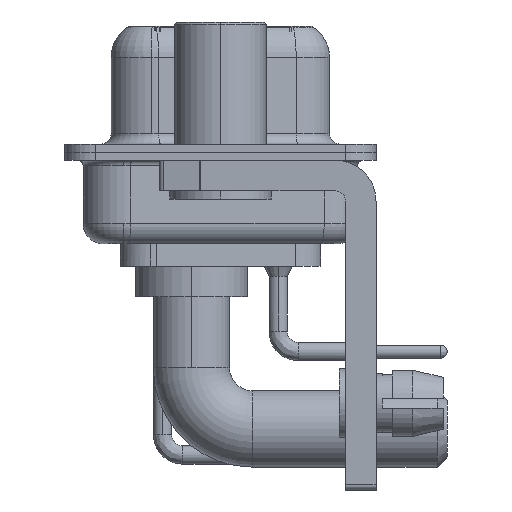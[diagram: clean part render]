
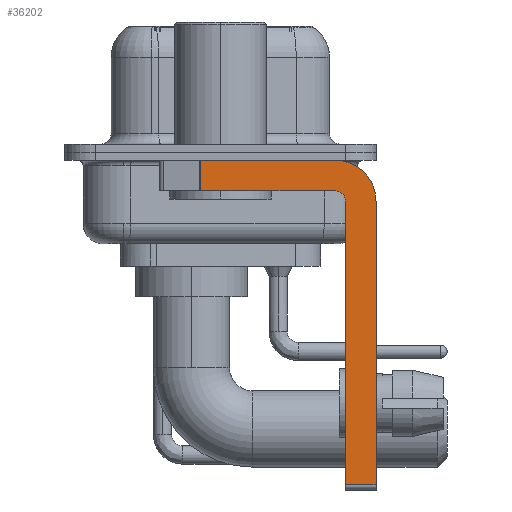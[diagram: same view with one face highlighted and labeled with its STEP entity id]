
A CAD part, left-side view. The second image highlights one B-rep face of the part: STEP entity #36202.
In plain terms, the highlighted planar face has unit normal (-1, 0, 0).
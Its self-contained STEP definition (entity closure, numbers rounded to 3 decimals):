
#147 = ORIENTED_EDGE ( 'NONE', *, *, #24818, .T. ) ;
#672 = VERTEX_POINT ( 'NONE', #22985 ) ;
#847 = DIRECTION ( 'NONE',  ( 0., -1., 0. ) ) ;
#1562 = VERTEX_POINT ( 'NONE', #23226 ) ;
#2220 = DIRECTION ( 'NONE',  ( 0., 0., -1. ) ) ;
#3119 = CARTESIAN_POINT ( 'NONE',  ( -2.9, -5.65, -2.4 ) ) ;
#3368 = CARTESIAN_POINT ( 'NONE',  ( -2.9, -7.65, -2.4 ) ) ;
#3698 = VECTOR ( 'NONE', #24557, 1000. ) ;
#4134 = EDGE_CURVE ( 'NONE', #32855, #33410, #8044, .T. ) ;
#4230 = LINE ( 'NONE', #33460, #3698 ) ;
#4348 = EDGE_CURVE ( 'NONE', #1562, #32855, #32166, .T. ) ;
#4890 = CARTESIAN_POINT ( 'NONE',  ( -2.9, -5.65, -2.4 ) ) ;
#5260 = DIRECTION ( 'NONE',  ( 1., 0., 0. ) ) ;
#5754 = LINE ( 'NONE', #34945, #12010 ) ;
#7094 = DIRECTION ( 'NONE',  ( 0., 0., -1. ) ) ;
#8044 = CIRCLE ( 'NONE', #25629, 2. ) ;
#8614 = EDGE_CURVE ( 'NONE', #25833, #672, #25494, .T. ) ;
#8709 = CARTESIAN_POINT ( 'NONE',  ( -2.9, -5.65, -16.35 ) ) ;
#8791 = DIRECTION ( 'NONE',  ( 0., 0., 1. ) ) ;
#9121 = AXIS2_PLACEMENT_3D ( 'NONE', #3119, #26480, #23445 ) ;
#9213 = CARTESIAN_POINT ( 'NONE',  ( -2.9, 3., -0.4 ) ) ;
#11501 = VECTOR ( 'NONE', #17260, 1000. ) ;
#12010 = VECTOR ( 'NONE', #8791, 1000. ) ;
#12273 = VECTOR ( 'NONE', #847, 1000. ) ;
#12539 = EDGE_LOOP ( 'NONE', ( #29477, #24041, #24917, #35046, #22544, #147, #31158, #20879 ) ) ;
#15218 = CARTESIAN_POINT ( 'NONE',  ( -2.9, -6.15, -2.4 ) ) ;
#15542 = CARTESIAN_POINT ( 'NONE',  ( -2.9, 0.978, -1.9 ) ) ;
#17131 = EDGE_CURVE ( 'NONE', #672, #18011, #26855, .T. ) ;
#17260 = DIRECTION ( 'NONE',  ( 0., -1., 0. ) ) ;
#17402 = EDGE_CURVE ( 'NONE', #26025, #25833, #5754, .T. ) ;
#18011 = VERTEX_POINT ( 'NONE', #15542 ) ;
#18676 = DIRECTION ( 'NONE',  ( 0., 1., 0. ) ) ;
#18722 = VERTEX_POINT ( 'NONE', #28975 ) ;
#19330 = CARTESIAN_POINT ( 'NONE',  ( -2.9, -5.65, -2.4 ) ) ;
#19875 = VECTOR ( 'NONE', #18676, 1000. ) ;
#20879 = ORIENTED_EDGE ( 'NONE', *, *, #4134, .F. ) ;
#21845 = AXIS2_PLACEMENT_3D ( 'NONE', #4890, #5260, #2220 ) ;
#22544 = ORIENTED_EDGE ( 'NONE', *, *, #17402, .F. ) ;
#22985 = CARTESIAN_POINT ( 'NONE',  ( -2.9, -5.65, -1.9 ) ) ;
#23226 = CARTESIAN_POINT ( 'NONE',  ( -2.9, 0.978, -0.4 ) ) ;
#23445 = DIRECTION ( 'NONE',  ( 0., 0., 1. ) ) ;
#23702 = LINE ( 'NONE', #8709, #11501 ) ;
#24041 = ORIENTED_EDGE ( 'NONE', *, *, #37238, .T. ) ;
#24557 = DIRECTION ( 'NONE',  ( 0., 0., -1. ) ) ;
#24818 = EDGE_CURVE ( 'NONE', #26025, #18722, #23702, .T. ) ;
#24917 = ORIENTED_EDGE ( 'NONE', *, *, #17131, .F. ) ;
#25494 = CIRCLE ( 'NONE', #9121, 0.5 ) ;
#25500 = CARTESIAN_POINT ( 'NONE',  ( -2.9, -5.65, -0.4 ) ) ;
#25629 = AXIS2_PLACEMENT_3D ( 'NONE', #19330, #34439, #36768 ) ;
#25833 = VERTEX_POINT ( 'NONE', #15218 ) ;
#26025 = VERTEX_POINT ( 'NONE', #33772 ) ;
#26480 = DIRECTION ( 'NONE',  ( -1., 0., 0. ) ) ;
#26855 = LINE ( 'NONE', #33094, #19875 ) ;
#27584 = LINE ( 'NONE', #33828, #35216 ) ;
#28975 = CARTESIAN_POINT ( 'NONE',  ( -2.9, -7.65, -16.35 ) ) ;
#29477 = ORIENTED_EDGE ( 'NONE', *, *, #4348, .F. ) ;
#31158 = ORIENTED_EDGE ( 'NONE', *, *, #37106, .F. ) ;
#32166 = LINE ( 'NONE', #9213, #12273 ) ;
#32855 = VERTEX_POINT ( 'NONE', #25500 ) ;
#33094 = CARTESIAN_POINT ( 'NONE',  ( -2.9, -5.65, -1.9 ) ) ;
#33361 = PLANE ( 'NONE',  #21845 ) ;
#33410 = VERTEX_POINT ( 'NONE', #3368 ) ;
#33460 = CARTESIAN_POINT ( 'NONE',  ( -2.9, -7.65, -2.4 ) ) ;
#33772 = CARTESIAN_POINT ( 'NONE',  ( -2.9, -6.15, -16.35 ) ) ;
#33828 = CARTESIAN_POINT ( 'NONE',  ( -2.9, 0.978, -1.9 ) ) ;
#34439 = DIRECTION ( 'NONE',  ( 1., 0., 0. ) ) ;
#34945 = CARTESIAN_POINT ( 'NONE',  ( -2.9, -6.15, -16.6 ) ) ;
#35046 = ORIENTED_EDGE ( 'NONE', *, *, #8614, .F. ) ;
#35216 = VECTOR ( 'NONE', #7094, 1000. ) ;
#36202 = ADVANCED_FACE ( 'NONE', ( #36933 ), #33361, .F. ) ;
#36768 = DIRECTION ( 'NONE',  ( 0., 0., -1. ) ) ;
#36933 = FACE_OUTER_BOUND ( 'NONE', #12539, .T. ) ;
#37106 = EDGE_CURVE ( 'NONE', #33410, #18722, #4230, .T. ) ;
#37238 = EDGE_CURVE ( 'NONE', #1562, #18011, #27584, .T. ) ;
